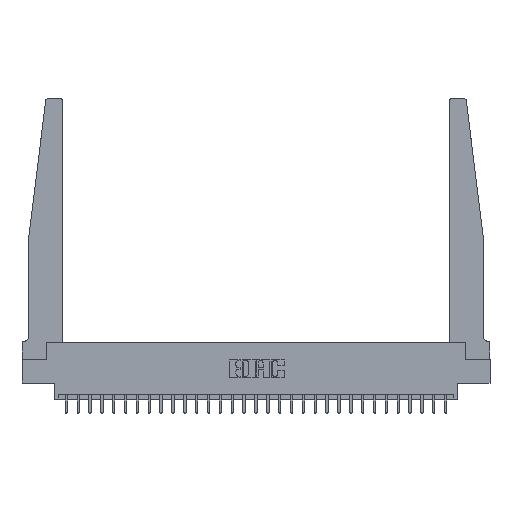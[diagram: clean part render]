
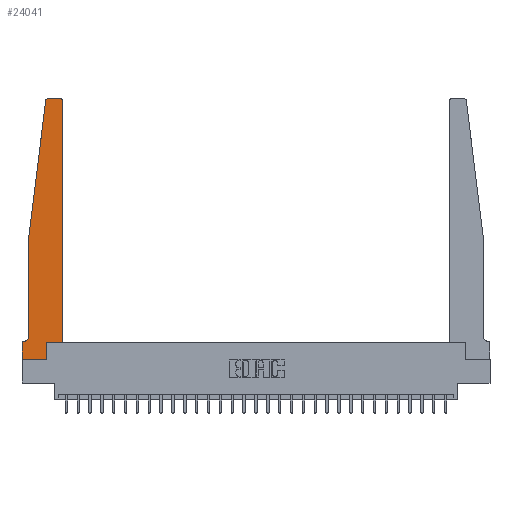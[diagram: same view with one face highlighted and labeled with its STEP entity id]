
A CAD part, top view. The second image highlights one B-rep face of the part: STEP entity #24041.
In plain terms, the highlighted planar face has unit normal (0, 0, 1).
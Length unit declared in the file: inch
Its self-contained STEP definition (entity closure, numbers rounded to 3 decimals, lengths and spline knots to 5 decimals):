
#309 = EDGE_CURVE ( 'NONE', #19218, #9827, #22918, .T. ) ;
#449 = LINE ( 'NONE', #13120, #11286 ) ;
#770 = CARTESIAN_POINT ( 'NONE',  ( 0.425, 0.18, 0.37 ) ) ;
#866 = CARTESIAN_POINT ( 'NONE',  ( 0.425, 2.72, 0.37 ) ) ;
#1109 = EDGE_CURVE ( 'NONE', #15108, #21543, #13502, .T. ) ;
#1150 = ORIENTED_EDGE ( 'NONE', *, *, #24512, .T. ) ;
#1394 = CARTESIAN_POINT ( 'NONE',  ( 0., 0.1875, 0.37 ) ) ;
#1534 = EDGE_CURVE ( 'NONE', #9827, #22096, #20523, .T. ) ;
#2530 = EDGE_CURVE ( 'NONE', #20804, #19218, #17219, .T. ) ;
#2898 = AXIS2_PLACEMENT_3D ( 'NONE', #7806, #22717, #9935 ) ;
#2969 = CIRCLE ( 'NONE', #2898, 0.03 ) ;
#3073 = LINE ( 'NONE', #10446, #25180 ) ;
#3346 = VECTOR ( 'NONE', #11614, 39.37008 ) ;
#3450 = DIRECTION ( 'NONE',  ( -1., 0., 0. ) ) ;
#4358 = EDGE_CURVE ( 'NONE', #26354, #8333, #2969, .T. ) ;
#5106 = LINE ( 'NONE', #7107, #15853 ) ;
#5181 = ORIENTED_EDGE ( 'NONE', *, *, #27029, .T. ) ;
#5499 = ORIENTED_EDGE ( 'NONE', *, *, #15024, .T. ) ;
#6240 = CARTESIAN_POINT ( 'NONE',  ( 0.015, 0.2375, 0.37 ) ) ;
#6311 = EDGE_CURVE ( 'NONE', #19053, #26354, #10025, .T. ) ;
#6686 = CARTESIAN_POINT ( 'NONE',  ( 0.395, 2.72, 0.37 ) ) ;
#6984 = ORIENTED_EDGE ( 'NONE', *, *, #16304, .T. ) ;
#7107 = CARTESIAN_POINT ( 'NONE',  ( 0.065, 0.1875, 0.37 ) ) ;
#7806 = CARTESIAN_POINT ( 'NONE',  ( 0.27653, 2.72, 0.37 ) ) ;
#8255 = DIRECTION ( 'NONE',  ( 0., -1., 0. ) ) ;
#8333 = VERTEX_POINT ( 'NONE', #12622 ) ;
#8428 = DIRECTION ( 'NONE',  ( -1., 0., 0. ) ) ;
#8542 = VECTOR ( 'NONE', #8255, 39.37008 ) ;
#8756 = ORIENTED_EDGE ( 'NONE', *, *, #11751, .T. ) ;
#8859 = DIRECTION ( 'NONE',  ( 1., 0., 0. ) ) ;
#8987 = CARTESIAN_POINT ( 'NONE',  ( 0.425, 0.18, 0.37 ) ) ;
#9178 = CARTESIAN_POINT ( 'NONE',  ( 0.2605, 0., 0.37 ) ) ;
#9587 = ORIENTED_EDGE ( 'NONE', *, *, #1109, .T. ) ;
#9827 = VERTEX_POINT ( 'NONE', #23390 ) ;
#9935 = DIRECTION ( 'NONE',  ( 1., 0., 0. ) ) ;
#10025 = LINE ( 'NONE', #24788, #15033 ) ;
#10183 = FACE_OUTER_BOUND ( 'NONE', #12740, .T. ) ;
#10446 = CARTESIAN_POINT ( 'NONE',  ( 0., 0., 0.37 ) ) ;
#11286 = VECTOR ( 'NONE', #15271, 39.37008 ) ;
#11560 = PLANE ( 'NONE',  #19963 ) ;
#11614 = DIRECTION ( 'NONE',  ( 1., 0., 0. ) ) ;
#11633 = ORIENTED_EDGE ( 'NONE', *, *, #22426, .T. ) ;
#11751 = EDGE_CURVE ( 'NONE', #21543, #26023, #19709, .T. ) ;
#12131 = CARTESIAN_POINT ( 'NONE',  ( 0., 0., 0.37 ) ) ;
#12446 = ORIENTED_EDGE ( 'NONE', *, *, #1534, .T. ) ;
#12536 = CARTESIAN_POINT ( 'NONE',  ( 0., 0., 0.37 ) ) ;
#12622 = CARTESIAN_POINT ( 'NONE',  ( 0.24675, 2.72367, 0.37 ) ) ;
#12740 = EDGE_LOOP ( 'NONE', ( #16869, #15254, #5181, #9587, #8756, #5499, #11633, #21188, #22574, #12446, #1150, #6984 ) ) ;
#12793 = CARTESIAN_POINT ( 'NONE',  ( 0.395, 2.75, 0.37 ) ) ;
#12812 = AXIS2_PLACEMENT_3D ( 'NONE', #6240, #21205, #8428 ) ;
#13120 = CARTESIAN_POINT ( 'NONE',  ( 0.065, 1.25, 0.37 ) ) ;
#13502 = LINE ( 'NONE', #21039, #8542 ) ;
#13741 = DIRECTION ( 'NONE',  ( 1., 0., 0. ) ) ;
#14698 = DIRECTION ( 'NONE',  ( 1., 0., 0. ) ) ;
#14914 = CARTESIAN_POINT ( 'NONE',  ( 0.2605, 0.18, 0.37 ) ) ;
#15024 = EDGE_CURVE ( 'NONE', #26023, #22992, #5106, .T. ) ;
#15033 = VECTOR ( 'NONE', #3450, 39.37008 ) ;
#15108 = VERTEX_POINT ( 'NONE', #22391 ) ;
#15129 = CARTESIAN_POINT ( 'NONE',  ( 0.27653, 2.75, 0.37 ) ) ;
#15162 = VECTOR ( 'NONE', #19703, 39.37008 ) ;
#15254 = ORIENTED_EDGE ( 'NONE', *, *, #4358, .T. ) ;
#15271 = DIRECTION ( 'NONE',  ( -0.122, -0.992, 0. ) ) ;
#15805 = CARTESIAN_POINT ( 'NONE',  ( 0., 0.1875, 0.37 ) ) ;
#15853 = VECTOR ( 'NONE', #26129, 39.37008 ) ;
#16304 = EDGE_CURVE ( 'NONE', #24051, #19053, #17872, .T. ) ;
#16869 = ORIENTED_EDGE ( 'NONE', *, *, #6311, .T. ) ;
#17184 = CARTESIAN_POINT ( 'NONE',  ( 0.065, 0.2375, 0.37 ) ) ;
#17195 = LINE ( 'NONE', #8987, #15162 ) ;
#17219 = LINE ( 'NONE', #12536, #22876 ) ;
#17872 = CIRCLE ( 'NONE', #23078, 0.03 ) ;
#19053 = VERTEX_POINT ( 'NONE', #12793 ) ;
#19218 = VERTEX_POINT ( 'NONE', #9178 ) ;
#19703 = DIRECTION ( 'NONE',  ( 0., 1., 0. ) ) ;
#19709 = CIRCLE ( 'NONE', #12812, 0.05 ) ;
#19963 = AXIS2_PLACEMENT_3D ( 'NONE', #15805, #26434, #13741 ) ;
#20385 = CARTESIAN_POINT ( 'NONE',  ( 0.015, 0.1875, 0.37 ) ) ;
#20523 = LINE ( 'NONE', #22290, #3346 ) ;
#20804 = VERTEX_POINT ( 'NONE', #12131 ) ;
#21039 = CARTESIAN_POINT ( 'NONE',  ( 0.065, 1.25, 0.37 ) ) ;
#21188 = ORIENTED_EDGE ( 'NONE', *, *, #2530, .T. ) ;
#21205 = DIRECTION ( 'NONE',  ( 0., 0., -1. ) ) ;
#21543 = VERTEX_POINT ( 'NONE', #17184 ) ;
#21620 = DIRECTION ( 'NONE',  ( 0., 0., 1. ) ) ;
#22096 = VERTEX_POINT ( 'NONE', #770 ) ;
#22290 = CARTESIAN_POINT ( 'NONE',  ( 0.425, 0.18, 0.37 ) ) ;
#22391 = CARTESIAN_POINT ( 'NONE',  ( 0.065, 1.25, 0.37 ) ) ;
#22426 = EDGE_CURVE ( 'NONE', #22992, #20804, #3073, .T. ) ;
#22574 = ORIENTED_EDGE ( 'NONE', *, *, #309, .T. ) ;
#22717 = DIRECTION ( 'NONE',  ( 0., 0., 1. ) ) ;
#22876 = VECTOR ( 'NONE', #14698, 39.37008 ) ;
#22918 = LINE ( 'NONE', #14914, #25816 ) ;
#22992 = VERTEX_POINT ( 'NONE', #1394 ) ;
#23078 = AXIS2_PLACEMENT_3D ( 'NONE', #6686, #21620, #8859 ) ;
#23390 = CARTESIAN_POINT ( 'NONE',  ( 0.2605, 0.18, 0.37 ) ) ;
#23435 = DIRECTION ( 'NONE',  ( 0., 1., 0. ) ) ;
#24041 = ADVANCED_FACE ( 'NONE', ( #10183 ), #11560, .T. ) ;
#24051 = VERTEX_POINT ( 'NONE', #866 ) ;
#24512 = EDGE_CURVE ( 'NONE', #22096, #24051, #17195, .T. ) ;
#24788 = CARTESIAN_POINT ( 'NONE',  ( 0.25, 2.75, 0.37 ) ) ;
#25180 = VECTOR ( 'NONE', #25303, 39.37008 ) ;
#25303 = DIRECTION ( 'NONE',  ( 0., -1., 0. ) ) ;
#25816 = VECTOR ( 'NONE', #23435, 39.37008 ) ;
#26023 = VERTEX_POINT ( 'NONE', #20385 ) ;
#26129 = DIRECTION ( 'NONE',  ( -1., 0., 0. ) ) ;
#26354 = VERTEX_POINT ( 'NONE', #15129 ) ;
#26434 = DIRECTION ( 'NONE',  ( 0., 0., 1. ) ) ;
#27029 = EDGE_CURVE ( 'NONE', #8333, #15108, #449, .T. ) ;
